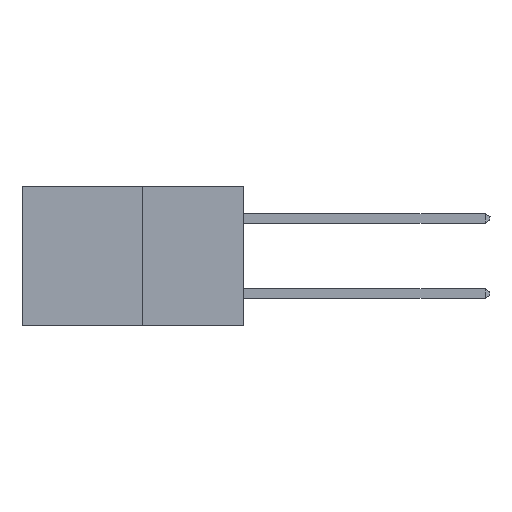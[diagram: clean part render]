
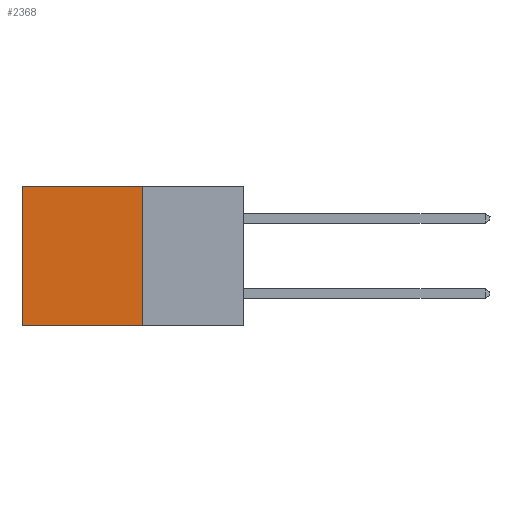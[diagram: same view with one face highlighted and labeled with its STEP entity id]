
A CAD part, left-side view. The second image highlights one B-rep face of the part: STEP entity #2368.
In plain terms, the highlighted planar face has unit normal (-1, 0, 0).
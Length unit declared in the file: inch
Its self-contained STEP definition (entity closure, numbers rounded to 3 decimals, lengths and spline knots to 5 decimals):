
#399 = EDGE_CURVE ( 'NONE', #4611, #1191, #7228, .T. ) ;
#438 = DIRECTION ( 'NONE',  ( 1., 0., 0. ) ) ;
#458 = DIRECTION ( 'NONE',  ( 0., 0., -1. ) ) ;
#515 = ORIENTED_EDGE ( 'NONE', *, *, #1899, .T. ) ;
#1191 = VERTEX_POINT ( 'NONE', #1289 ) ;
#1289 = CARTESIAN_POINT ( 'NONE',  ( 0.277, 0.59, -0.37 ) ) ;
#1588 = DIRECTION ( 'NONE',  ( 0., 1., 0. ) ) ;
#1609 = FACE_OUTER_BOUND ( 'NONE', #8752, .T. ) ;
#1899 = EDGE_CURVE ( 'NONE', #2652, #4611, #2134, .T. ) ;
#1983 = CARTESIAN_POINT ( 'NONE',  ( 0.277, 0.27, 0. ) ) ;
#2043 = CARTESIAN_POINT ( 'NONE',  ( 0.277, 0.27, -0.37 ) ) ;
#2134 = LINE ( 'NONE', #5238, #7493 ) ;
#2318 = CARTESIAN_POINT ( 'NONE',  ( 0.277, 0.27, -0.37 ) ) ;
#2368 = ADVANCED_FACE ( 'NONE', ( #1609 ), #6296, .F. ) ;
#2652 = VERTEX_POINT ( 'NONE', #1983 ) ;
#2696 = ORIENTED_EDGE ( 'NONE', *, *, #4655, .F. ) ;
#2735 = DIRECTION ( 'NONE',  ( 0., 0., -1. ) ) ;
#3236 = CARTESIAN_POINT ( 'NONE',  ( 0.277, 0.27, -0.37 ) ) ;
#3384 = VECTOR ( 'NONE', #9436, 39.37008 ) ;
#3673 = VECTOR ( 'NONE', #4099, 39.37008 ) ;
#4099 = DIRECTION ( 'NONE',  ( 0., 0., -1. ) ) ;
#4139 = LINE ( 'NONE', #2043, #9260 ) ;
#4611 = VERTEX_POINT ( 'NONE', #5108 ) ;
#4655 = EDGE_CURVE ( 'NONE', #5837, #1191, #7165, .T. ) ;
#4831 = EDGE_CURVE ( 'NONE', #2652, #5837, #4139, .T. ) ;
#5108 = CARTESIAN_POINT ( 'NONE',  ( 0.277, 0.59, 0. ) ) ;
#5238 = CARTESIAN_POINT ( 'NONE',  ( 0.277, 0.27, 0. ) ) ;
#5821 = AXIS2_PLACEMENT_3D ( 'NONE', #3236, #438, #2735 ) ;
#5837 = VERTEX_POINT ( 'NONE', #2318 ) ;
#6234 = ORIENTED_EDGE ( 'NONE', *, *, #4831, .F. ) ;
#6296 = PLANE ( 'NONE',  #5821 ) ;
#6469 = CARTESIAN_POINT ( 'NONE',  ( 0.277, 0.27, -0.37 ) ) ;
#7165 = LINE ( 'NONE', #6469, #3384 ) ;
#7228 = LINE ( 'NONE', #8163, #3673 ) ;
#7352 = ORIENTED_EDGE ( 'NONE', *, *, #399, .T. ) ;
#7493 = VECTOR ( 'NONE', #1588, 39.37008 ) ;
#8163 = CARTESIAN_POINT ( 'NONE',  ( 0.277, 0.59, -0.37 ) ) ;
#8752 = EDGE_LOOP ( 'NONE', ( #7352, #2696, #6234, #515 ) ) ;
#9260 = VECTOR ( 'NONE', #458, 39.37008 ) ;
#9436 = DIRECTION ( 'NONE',  ( 0., 1., 0. ) ) ;
